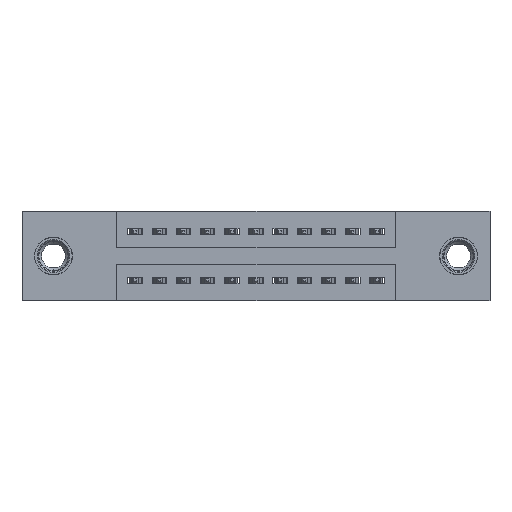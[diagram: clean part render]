
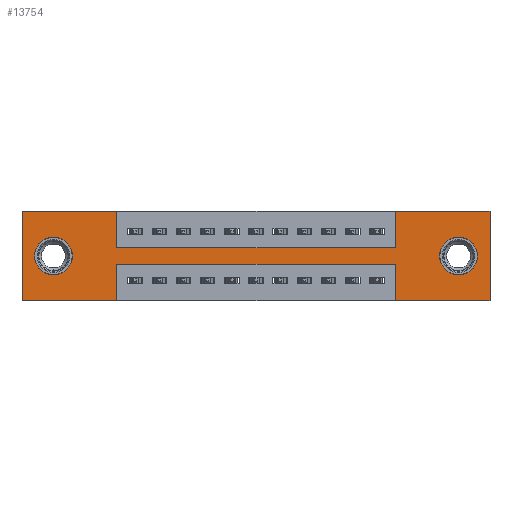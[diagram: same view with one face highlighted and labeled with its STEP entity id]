
A CAD part, front view. The second image highlights one B-rep face of the part: STEP entity #13754.
In plain terms, the highlighted planar face has unit normal (0, -1, 0).
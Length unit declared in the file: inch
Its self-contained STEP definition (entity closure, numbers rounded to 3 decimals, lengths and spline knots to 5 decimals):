
#116 = LINE ( 'NONE', #866, #11341 ) ;
#332 = CARTESIAN_POINT ( 'NONE',  ( 1.805, 0., -0.107 ) ) ;
#335 = ORIENTED_EDGE ( 'NONE', *, *, #5432, .T. ) ;
#492 = ORIENTED_EDGE ( 'NONE', *, *, #11122, .T. ) ;
#702 = LINE ( 'NONE', #5972, #5831 ) ;
#727 = CARTESIAN_POINT ( 'NONE',  ( 1.805, 0., -0.263 ) ) ;
#866 = CARTESIAN_POINT ( 'NONE',  ( 0., 0., 0. ) ) ;
#928 = ORIENTED_EDGE ( 'NONE', *, *, #13747, .F. ) ;
#1037 = DIRECTION ( 'NONE',  ( -1., 0., 0. ) ) ;
#1141 = VERTEX_POINT ( 'NONE', #6569 ) ;
#1152 = CARTESIAN_POINT ( 'NONE',  ( 0.3925, 0., -0.22 ) ) ;
#1168 = VERTEX_POINT ( 'NONE', #7976 ) ;
#1253 = CARTESIAN_POINT ( 'NONE',  ( 0., 0., -0.37 ) ) ;
#1281 = VERTEX_POINT ( 'NONE', #5645 ) ;
#1299 = DIRECTION ( 'NONE',  ( 0., 0., -1. ) ) ;
#1795 = ORIENTED_EDGE ( 'NONE', *, *, #8021, .T. ) ;
#1801 = CARTESIAN_POINT ( 'NONE',  ( 1.805, 0., -0.185 ) ) ;
#2029 = ORIENTED_EDGE ( 'NONE', *, *, #8401, .T. ) ;
#2088 = EDGE_CURVE ( 'NONE', #12862, #12388, #10057, .T. ) ;
#2188 = EDGE_CURVE ( 'NONE', #7964, #13897, #702, .T. ) ;
#2291 = AXIS2_PLACEMENT_3D ( 'NONE', #9954, #7882, #1299 ) ;
#2524 = ORIENTED_EDGE ( 'NONE', *, *, #10524, .F. ) ;
#2526 = DIRECTION ( 'NONE',  ( 0., 0., -1. ) ) ;
#2527 = VECTOR ( 'NONE', #4188, 39.37008 ) ;
#2650 = EDGE_CURVE ( 'NONE', #13897, #2896, #13014, .T. ) ;
#2688 = DIRECTION ( 'NONE',  ( 0., 1., 0. ) ) ;
#2877 = LINE ( 'NONE', #3081, #2527 ) ;
#2896 = VERTEX_POINT ( 'NONE', #12321 ) ;
#2904 = DIRECTION ( 'NONE',  ( 0., 0., -1. ) ) ;
#2931 = ORIENTED_EDGE ( 'NONE', *, *, #6056, .F. ) ;
#2954 = LINE ( 'NONE', #1253, #8457 ) ;
#3009 = ORIENTED_EDGE ( 'NONE', *, *, #4115, .F. ) ;
#3081 = CARTESIAN_POINT ( 'NONE',  ( 0., 0., 0. ) ) ;
#3117 = VERTEX_POINT ( 'NONE', #727 ) ;
#3459 = DIRECTION ( 'NONE',  ( -1., 0., 0. ) ) ;
#3464 = EDGE_LOOP ( 'NONE', ( #492, #2029 ) ) ;
#3654 = AXIS2_PLACEMENT_3D ( 'NONE', #9241, #2688, #10299 ) ;
#3693 = ORIENTED_EDGE ( 'NONE', *, *, #10498, .F. ) ;
#3801 = ORIENTED_EDGE ( 'NONE', *, *, #2088, .F. ) ;
#3834 = DIRECTION ( 'NONE',  ( 0., 0., -1. ) ) ;
#3931 = CARTESIAN_POINT ( 'NONE',  ( 0.3925, 0., -0.37 ) ) ;
#4110 = VECTOR ( 'NONE', #3834, 39.37008 ) ;
#4115 = EDGE_CURVE ( 'NONE', #12388, #1168, #12706, .T. ) ;
#4188 = DIRECTION ( 'NONE',  ( 0., 0., 1. ) ) ;
#4190 = VERTEX_POINT ( 'NONE', #3931 ) ;
#4210 = VERTEX_POINT ( 'NONE', #10481 ) ;
#4391 = VERTEX_POINT ( 'NONE', #7579 ) ;
#4673 = VERTEX_POINT ( 'NONE', #332 ) ;
#4751 = EDGE_LOOP ( 'NONE', ( #335, #1795 ) ) ;
#4890 = CIRCLE ( 'NONE', #10400, 0.078 ) ;
#4914 = ORIENTED_EDGE ( 'NONE', *, *, #11223, .F. ) ;
#5158 = CARTESIAN_POINT ( 'NONE',  ( 0., 0., -0.37 ) ) ;
#5224 = CARTESIAN_POINT ( 'NONE',  ( 1.5425, 0., 0. ) ) ;
#5258 = LINE ( 'NONE', #13757, #13491 ) ;
#5432 = EDGE_CURVE ( 'NONE', #8120, #1141, #13660, .T. ) ;
#5518 = FACE_BOUND ( 'NONE', #4751, .T. ) ;
#5584 = CARTESIAN_POINT ( 'NONE',  ( 1.935, 0., 0. ) ) ;
#5645 = CARTESIAN_POINT ( 'NONE',  ( 1.5425, 0., -0.15 ) ) ;
#5690 = EDGE_CURVE ( 'NONE', #9424, #1281, #5258, .T. ) ;
#5719 = VECTOR ( 'NONE', #9020, 39.37008 ) ;
#5831 = VECTOR ( 'NONE', #6052, 39.37008 ) ;
#5857 = DIRECTION ( 'NONE',  ( 0., 1., 0. ) ) ;
#5867 = FACE_BOUND ( 'NONE', #3464, .T. ) ;
#5946 = VECTOR ( 'NONE', #2526, 39.37008 ) ;
#5972 = CARTESIAN_POINT ( 'NONE',  ( 1.5425, 0., -0.37 ) ) ;
#6052 = DIRECTION ( 'NONE',  ( 0., 0., 1. ) ) ;
#6056 = EDGE_CURVE ( 'NONE', #2896, #4190, #6276, .T. ) ;
#6058 = AXIS2_PLACEMENT_3D ( 'NONE', #6286, #13770, #7414 ) ;
#6172 = CARTESIAN_POINT ( 'NONE',  ( 1.5425, 0., 0. ) ) ;
#6276 = LINE ( 'NONE', #6957, #5946 ) ;
#6286 = CARTESIAN_POINT ( 'NONE',  ( 0.13, 0., -0.185 ) ) ;
#6344 = DIRECTION ( 'NONE',  ( 1., 0., 0. ) ) ;
#6517 = VERTEX_POINT ( 'NONE', #13391 ) ;
#6569 = CARTESIAN_POINT ( 'NONE',  ( 0.13, 0., -0.263 ) ) ;
#6746 = PLANE ( 'NONE',  #2291 ) ;
#6822 = CARTESIAN_POINT ( 'NONE',  ( 0.3925, 0., 0. ) ) ;
#6848 = ORIENTED_EDGE ( 'NONE', *, *, #9942, .F. ) ;
#6867 = VECTOR ( 'NONE', #6933, 39.37008 ) ;
#6933 = DIRECTION ( 'NONE',  ( 1., 0., 0. ) ) ;
#6949 = CARTESIAN_POINT ( 'NONE',  ( 0., 0., 0. ) ) ;
#6957 = CARTESIAN_POINT ( 'NONE',  ( 0.3925, 0., -0.37 ) ) ;
#7319 = CARTESIAN_POINT ( 'NONE',  ( 1.5425, 0., -0.37 ) ) ;
#7414 = DIRECTION ( 'NONE',  ( 0., 0., 1. ) ) ;
#7579 = CARTESIAN_POINT ( 'NONE',  ( 0.3925, 0., 0. ) ) ;
#7882 = DIRECTION ( 'NONE',  ( 0., -1., 0. ) ) ;
#7964 = VERTEX_POINT ( 'NONE', #7319 ) ;
#7976 = CARTESIAN_POINT ( 'NONE',  ( 1.935, 0., -0.37 ) ) ;
#8021 = EDGE_CURVE ( 'NONE', #1141, #8120, #13419, .T. ) ;
#8120 = VERTEX_POINT ( 'NONE', #12846 ) ;
#8401 = EDGE_CURVE ( 'NONE', #3117, #4673, #11265, .T. ) ;
#8457 = VECTOR ( 'NONE', #3459, 39.37008 ) ;
#9020 = DIRECTION ( 'NONE',  ( 0., 0., -1. ) ) ;
#9170 = EDGE_LOOP ( 'NONE', ( #2931, #11773, #12834, #928, #3009, #3801, #3693, #13000, #10302, #4914, #6848, #2524 ) ) ;
#9191 = VECTOR ( 'NONE', #11624, 39.37008 ) ;
#9241 = CARTESIAN_POINT ( 'NONE',  ( 0.13, 0., -0.185 ) ) ;
#9424 = VERTEX_POINT ( 'NONE', #12803 ) ;
#9434 = DIRECTION ( 'NONE',  ( 0., 1., 0. ) ) ;
#9509 = VECTOR ( 'NONE', #10537, 39.37008 ) ;
#9942 = EDGE_CURVE ( 'NONE', #4210, #6517, #2877, .T. ) ;
#9954 = CARTESIAN_POINT ( 'NONE',  ( 0., 0., -0.37 ) ) ;
#10057 = LINE ( 'NONE', #6949, #6867 ) ;
#10140 = AXIS2_PLACEMENT_3D ( 'NONE', #12277, #5857, #13343 ) ;
#10207 = VECTOR ( 'NONE', #1037, 39.37008 ) ;
#10299 = DIRECTION ( 'NONE',  ( 0., 0., 1. ) ) ;
#10302 = ORIENTED_EDGE ( 'NONE', *, *, #13135, .F. ) ;
#10400 = AXIS2_PLACEMENT_3D ( 'NONE', #1801, #9434, #2904 ) ;
#10481 = CARTESIAN_POINT ( 'NONE',  ( 0., 0., -0.37 ) ) ;
#10498 = EDGE_CURVE ( 'NONE', #1281, #12862, #12319, .T. ) ;
#10524 = EDGE_CURVE ( 'NONE', #4190, #4210, #11991, .T. ) ;
#10537 = DIRECTION ( 'NONE',  ( 0., 0., 1. ) ) ;
#11122 = EDGE_CURVE ( 'NONE', #4673, #3117, #4890, .T. ) ;
#11223 = EDGE_CURVE ( 'NONE', #6517, #4391, #116, .T. ) ;
#11265 = CIRCLE ( 'NONE', #10140, 0.078 ) ;
#11341 = VECTOR ( 'NONE', #6344, 39.37008 ) ;
#11352 = CARTESIAN_POINT ( 'NONE',  ( 1.935, 0., 0. ) ) ;
#11437 = LINE ( 'NONE', #6822, #5719 ) ;
#11624 = DIRECTION ( 'NONE',  ( -1., 0., 0. ) ) ;
#11773 = ORIENTED_EDGE ( 'NONE', *, *, #2650, .F. ) ;
#11991 = LINE ( 'NONE', #5158, #9191 ) ;
#12277 = CARTESIAN_POINT ( 'NONE',  ( 1.805, 0., -0.185 ) ) ;
#12319 = LINE ( 'NONE', #6172, #9509 ) ;
#12321 = CARTESIAN_POINT ( 'NONE',  ( 0.3925, 0., -0.22 ) ) ;
#12388 = VERTEX_POINT ( 'NONE', #5584 ) ;
#12649 = DIRECTION ( 'NONE',  ( 1., 0., 0. ) ) ;
#12706 = LINE ( 'NONE', #11352, #4110 ) ;
#12803 = CARTESIAN_POINT ( 'NONE',  ( 0.3925, 0., -0.15 ) ) ;
#12834 = ORIENTED_EDGE ( 'NONE', *, *, #2188, .F. ) ;
#12846 = CARTESIAN_POINT ( 'NONE',  ( 0.13, 0., -0.107 ) ) ;
#12862 = VERTEX_POINT ( 'NONE', #5224 ) ;
#13000 = ORIENTED_EDGE ( 'NONE', *, *, #5690, .F. ) ;
#13014 = LINE ( 'NONE', #1152, #10207 ) ;
#13135 = EDGE_CURVE ( 'NONE', #4391, #9424, #11437, .T. ) ;
#13343 = DIRECTION ( 'NONE',  ( 0., 0., -1. ) ) ;
#13391 = CARTESIAN_POINT ( 'NONE',  ( 0., 0., 0. ) ) ;
#13414 = CARTESIAN_POINT ( 'NONE',  ( 1.5425, 0., -0.22 ) ) ;
#13419 = CIRCLE ( 'NONE', #6058, 0.078 ) ;
#13491 = VECTOR ( 'NONE', #12649, 39.37008 ) ;
#13660 = CIRCLE ( 'NONE', #3654, 0.078 ) ;
#13733 = FACE_OUTER_BOUND ( 'NONE', #9170, .T. ) ;
#13747 = EDGE_CURVE ( 'NONE', #1168, #7964, #2954, .T. ) ;
#13754 = ADVANCED_FACE ( 'NONE', ( #5867, #5518, #13733 ), #6746, .T. ) ;
#13757 = CARTESIAN_POINT ( 'NONE',  ( 0.3925, 0., -0.15 ) ) ;
#13770 = DIRECTION ( 'NONE',  ( 0., 1., 0. ) ) ;
#13897 = VERTEX_POINT ( 'NONE', #13414 ) ;
